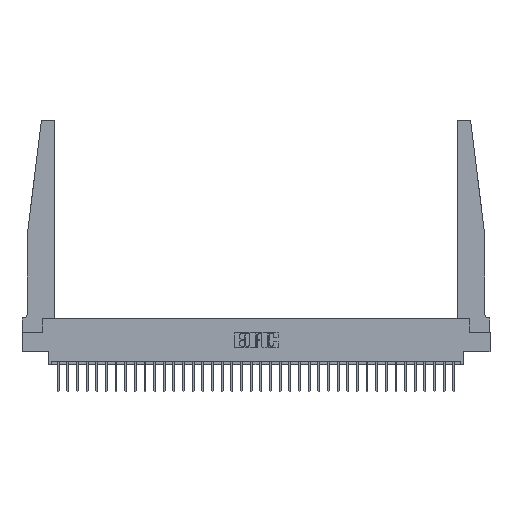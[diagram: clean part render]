
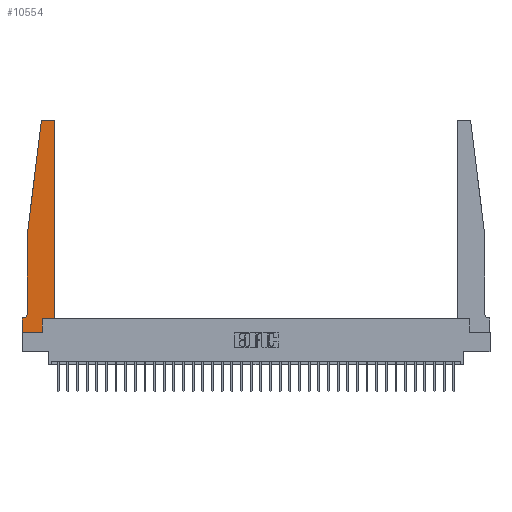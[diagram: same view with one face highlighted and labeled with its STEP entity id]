
A CAD part, top view. The second image highlights one B-rep face of the part: STEP entity #10554.
In plain terms, the highlighted planar face has unit normal (0, 0, 1).
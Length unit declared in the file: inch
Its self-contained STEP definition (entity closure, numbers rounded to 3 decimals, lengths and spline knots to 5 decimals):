
#1119 = CARTESIAN_POINT ( 'NONE',  ( 0.2605, 0.18, 0.37 ) ) ;
#1172 = CARTESIAN_POINT ( 'NONE',  ( 0., 0., 0.37 ) ) ;
#1266 = DIRECTION ( 'NONE',  ( 0., 0., -1. ) ) ;
#1594 = VERTEX_POINT ( 'NONE', #26946 ) ;
#2149 = DIRECTION ( 'NONE',  ( 1., 0., 0. ) ) ;
#2185 = VERTEX_POINT ( 'NONE', #27228 ) ;
#3009 = CARTESIAN_POINT ( 'NONE',  ( 0.25, 2.75, 0.37 ) ) ;
#3131 = DIRECTION ( 'NONE',  ( 0., 1., 0. ) ) ;
#3908 = DIRECTION ( 'NONE',  ( 0., 1., 0. ) ) ;
#4111 = VERTEX_POINT ( 'NONE', #1119 ) ;
#4127 = CIRCLE ( 'NONE', #21608, 0.03 ) ;
#4254 = ORIENTED_EDGE ( 'NONE', *, *, #30652, .T. ) ;
#4345 = DIRECTION ( 'NONE',  ( -1., 0., 0. ) ) ;
#4401 = LINE ( 'NONE', #24618, #18638 ) ;
#4553 = VECTOR ( 'NONE', #15944, 39.37008 ) ;
#5055 = LINE ( 'NONE', #22622, #15004 ) ;
#5422 = VERTEX_POINT ( 'NONE', #30307 ) ;
#5558 = ORIENTED_EDGE ( 'NONE', *, *, #28712, .T. ) ;
#5655 = DIRECTION ( 'NONE',  ( 1., 0., 0. ) ) ;
#5833 = VECTOR ( 'NONE', #5655, 39.37008 ) ;
#7138 = DIRECTION ( 'NONE',  ( 0., 0., 1. ) ) ;
#7630 = DIRECTION ( 'NONE',  ( 1., 0., 0. ) ) ;
#7722 = EDGE_CURVE ( 'NONE', #22601, #14528, #28065, .T. ) ;
#7783 = CARTESIAN_POINT ( 'NONE',  ( 0.395, 2.72, 0.37 ) ) ;
#9664 = CARTESIAN_POINT ( 'NONE',  ( 0.065, 0.2375, 0.37 ) ) ;
#9861 = EDGE_CURVE ( 'NONE', #16616, #12277, #25296, .T. ) ;
#10554 = ADVANCED_FACE ( 'NONE', ( #30210 ), #30366, .T. ) ;
#10685 = CARTESIAN_POINT ( 'NONE',  ( 0.27653, 2.72, 0.37 ) ) ;
#10885 = VERTEX_POINT ( 'NONE', #15220 ) ;
#11482 = LINE ( 'NONE', #31748, #12206 ) ;
#12049 = AXIS2_PLACEMENT_3D ( 'NONE', #7783, #27862, #28033 ) ;
#12206 = VECTOR ( 'NONE', #19616, 39.37008 ) ;
#12277 = VERTEX_POINT ( 'NONE', #27838 ) ;
#12349 = DIRECTION ( 'NONE',  ( -0.122, -0.992, 0. ) ) ;
#13067 = EDGE_CURVE ( 'NONE', #1594, #4111, #13232, .T. ) ;
#13232 = LINE ( 'NONE', #20541, #14317 ) ;
#13334 = DIRECTION ( 'NONE',  ( 1., 0., 0. ) ) ;
#13342 = VECTOR ( 'NONE', #25056, 39.37008 ) ;
#13461 = ORIENTED_EDGE ( 'NONE', *, *, #13067, .T. ) ;
#13824 = EDGE_CURVE ( 'NONE', #5422, #16616, #11482, .T. ) ;
#14057 = ORIENTED_EDGE ( 'NONE', *, *, #13824, .T. ) ;
#14317 = VECTOR ( 'NONE', #3131, 39.37008 ) ;
#14528 = VERTEX_POINT ( 'NONE', #20868 ) ;
#14602 = CARTESIAN_POINT ( 'NONE',  ( 0.065, 0.1875, 0.37 ) ) ;
#14737 = CARTESIAN_POINT ( 'NONE',  ( 0.425, 0.18, 0.37 ) ) ;
#15004 = VECTOR ( 'NONE', #12349, 39.37008 ) ;
#15091 = CARTESIAN_POINT ( 'NONE',  ( 0., 0.1875, 0.37 ) ) ;
#15160 = EDGE_LOOP ( 'NONE', ( #32748, #29293, #25242, #14057, #32648, #25888, #5558, #25829, #13461, #17564, #4254, #21248 ) ) ;
#15220 = CARTESIAN_POINT ( 'NONE',  ( 0.425, 0.18, 0.37 ) ) ;
#15944 = DIRECTION ( 'NONE',  ( -1., 0., 0. ) ) ;
#16280 = AXIS2_PLACEMENT_3D ( 'NONE', #26152, #1266, #31318 ) ;
#16616 = VERTEX_POINT ( 'NONE', #9664 ) ;
#17564 = ORIENTED_EDGE ( 'NONE', *, *, #25118, .T. ) ;
#18451 = EDGE_CURVE ( 'NONE', #12277, #32331, #22064, .T. ) ;
#18638 = VECTOR ( 'NONE', #3908, 39.37008 ) ;
#19616 = DIRECTION ( 'NONE',  ( 0., -1., 0. ) ) ;
#20014 = CIRCLE ( 'NONE', #12049, 0.03 ) ;
#20252 = CARTESIAN_POINT ( 'NONE',  ( 0., 0., 0.37 ) ) ;
#20541 = CARTESIAN_POINT ( 'NONE',  ( 0.2605, 0.18, 0.37 ) ) ;
#20597 = VECTOR ( 'NONE', #2149, 39.37008 ) ;
#20868 = CARTESIAN_POINT ( 'NONE',  ( 0.27653, 2.75, 0.37 ) ) ;
#21248 = ORIENTED_EDGE ( 'NONE', *, *, #23572, .T. ) ;
#21608 = AXIS2_PLACEMENT_3D ( 'NONE', #10685, #26272, #13334 ) ;
#22064 = LINE ( 'NONE', #14602, #24529 ) ;
#22601 = VERTEX_POINT ( 'NONE', #28982 ) ;
#22622 = CARTESIAN_POINT ( 'NONE',  ( 0.065, 1.25, 0.37 ) ) ;
#23572 = EDGE_CURVE ( 'NONE', #2185, #22601, #20014, .T. ) ;
#23666 = VERTEX_POINT ( 'NONE', #25862 ) ;
#23986 = EDGE_CURVE ( 'NONE', #14528, #23666, #4127, .T. ) ;
#24098 = CARTESIAN_POINT ( 'NONE',  ( 0., 0., 0.37 ) ) ;
#24529 = VECTOR ( 'NONE', #4345, 39.37008 ) ;
#24618 = CARTESIAN_POINT ( 'NONE',  ( 0.425, 0.18, 0.37 ) ) ;
#25056 = DIRECTION ( 'NONE',  ( 0., -1., 0. ) ) ;
#25118 = EDGE_CURVE ( 'NONE', #4111, #10885, #32671, .T. ) ;
#25242 = ORIENTED_EDGE ( 'NONE', *, *, #32190, .T. ) ;
#25296 = CIRCLE ( 'NONE', #16280, 0.05 ) ;
#25388 = LINE ( 'NONE', #20252, #13342 ) ;
#25829 = ORIENTED_EDGE ( 'NONE', *, *, #26015, .T. ) ;
#25862 = CARTESIAN_POINT ( 'NONE',  ( 0.24675, 2.72367, 0.37 ) ) ;
#25888 = ORIENTED_EDGE ( 'NONE', *, *, #18451, .T. ) ;
#26015 = EDGE_CURVE ( 'NONE', #27557, #1594, #28566, .T. ) ;
#26152 = CARTESIAN_POINT ( 'NONE',  ( 0.015, 0.2375, 0.37 ) ) ;
#26272 = DIRECTION ( 'NONE',  ( 0., 0., 1. ) ) ;
#26946 = CARTESIAN_POINT ( 'NONE',  ( 0.2605, 0., 0.37 ) ) ;
#27228 = CARTESIAN_POINT ( 'NONE',  ( 0.425, 2.72, 0.37 ) ) ;
#27557 = VERTEX_POINT ( 'NONE', #24098 ) ;
#27838 = CARTESIAN_POINT ( 'NONE',  ( 0.015, 0.1875, 0.37 ) ) ;
#27862 = DIRECTION ( 'NONE',  ( 0., 0., 1. ) ) ;
#28033 = DIRECTION ( 'NONE',  ( 1., 0., 0. ) ) ;
#28065 = LINE ( 'NONE', #3009, #4553 ) ;
#28269 = CARTESIAN_POINT ( 'NONE',  ( 0., 0.1875, 0.37 ) ) ;
#28566 = LINE ( 'NONE', #1172, #5833 ) ;
#28712 = EDGE_CURVE ( 'NONE', #32331, #27557, #25388, .T. ) ;
#28982 = CARTESIAN_POINT ( 'NONE',  ( 0.395, 2.75, 0.37 ) ) ;
#29293 = ORIENTED_EDGE ( 'NONE', *, *, #23986, .T. ) ;
#29582 = AXIS2_PLACEMENT_3D ( 'NONE', #15091, #7138, #7630 ) ;
#30210 = FACE_OUTER_BOUND ( 'NONE', #15160, .T. ) ;
#30307 = CARTESIAN_POINT ( 'NONE',  ( 0.065, 1.25, 0.37 ) ) ;
#30366 = PLANE ( 'NONE',  #29582 ) ;
#30652 = EDGE_CURVE ( 'NONE', #10885, #2185, #4401, .T. ) ;
#31318 = DIRECTION ( 'NONE',  ( -1., 0., 0. ) ) ;
#31748 = CARTESIAN_POINT ( 'NONE',  ( 0.065, 1.25, 0.37 ) ) ;
#32190 = EDGE_CURVE ( 'NONE', #23666, #5422, #5055, .T. ) ;
#32331 = VERTEX_POINT ( 'NONE', #28269 ) ;
#32648 = ORIENTED_EDGE ( 'NONE', *, *, #9861, .T. ) ;
#32671 = LINE ( 'NONE', #14737, #20597 ) ;
#32748 = ORIENTED_EDGE ( 'NONE', *, *, #7722, .T. ) ;
